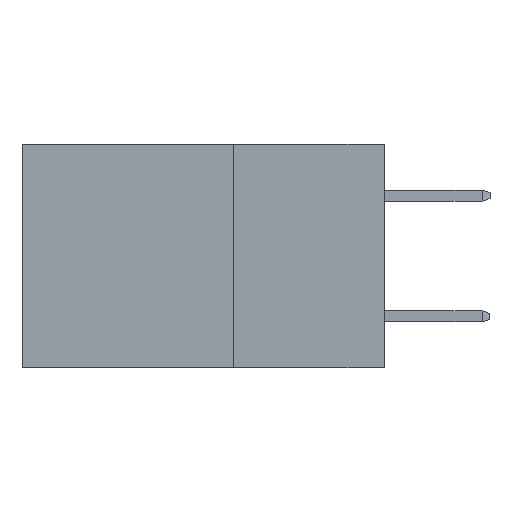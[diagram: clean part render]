
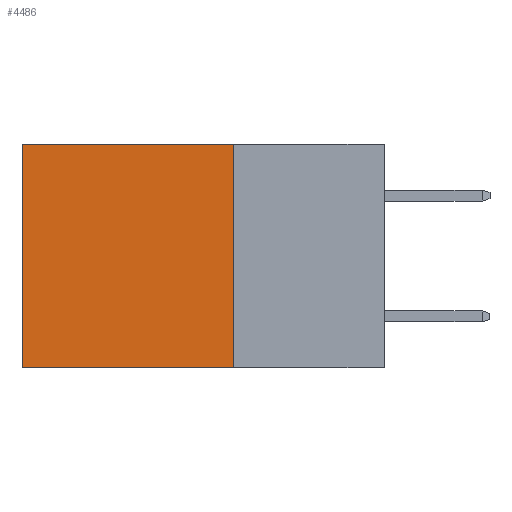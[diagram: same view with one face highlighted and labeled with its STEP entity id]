
A CAD part, left-side view. The second image highlights one B-rep face of the part: STEP entity #4486.
In plain terms, the highlighted planar face has unit normal (-1, 0, 0).
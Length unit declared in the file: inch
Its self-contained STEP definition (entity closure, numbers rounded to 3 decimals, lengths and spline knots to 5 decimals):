
#192 = LINE ( 'NONE', #7564, #5779 ) ;
#226 = VERTEX_POINT ( 'NONE', #15000 ) ;
#318 = LINE ( 'NONE', #11781, #12162 ) ;
#362 = ORIENTED_EDGE ( 'NONE', *, *, #3451, .F. ) ;
#821 = ORIENTED_EDGE ( 'NONE', *, *, #5099, .T. ) ;
#1122 = AXIS2_PLACEMENT_3D ( 'NONE', #11481, #11484, #8219 ) ;
#1388 = CARTESIAN_POINT ( 'NONE',  ( 0.298, 0.6, -0.37 ) ) ;
#1600 = DIRECTION ( 'NONE',  ( 0., 0., -1. ) ) ;
#1629 = DIRECTION ( 'NONE',  ( 0., 1., 0. ) ) ;
#2993 = VERTEX_POINT ( 'NONE', #5048 ) ;
#3451 = EDGE_CURVE ( 'NONE', #226, #10245, #6701, .T. ) ;
#4212 = FACE_OUTER_BOUND ( 'NONE', #6698, .T. ) ;
#4276 = ORIENTED_EDGE ( 'NONE', *, *, #15210, .T. ) ;
#4344 = CARTESIAN_POINT ( 'NONE',  ( 0.298, 0.6, 0. ) ) ;
#4486 = ADVANCED_FACE ( 'NONE', ( #4212 ), #12796, .F. ) ;
#5048 = CARTESIAN_POINT ( 'NONE',  ( 0.298, 0.25, 0. ) ) ;
#5099 = EDGE_CURVE ( 'NONE', #2993, #13568, #318, .T. ) ;
#5779 = VECTOR ( 'NONE', #1600, 39.37008 ) ;
#6698 = EDGE_LOOP ( 'NONE', ( #4276, #362, #14843, #821 ) ) ;
#6701 = LINE ( 'NONE', #14735, #9824 ) ;
#7564 = CARTESIAN_POINT ( 'NONE',  ( 0.298, 0.6, 0. ) ) ;
#7876 = VECTOR ( 'NONE', #12480, 39.37008 ) ;
#8219 = DIRECTION ( 'NONE',  ( 0., 0., -1. ) ) ;
#8327 = EDGE_CURVE ( 'NONE', #2993, #226, #14438, .T. ) ;
#9824 = VECTOR ( 'NONE', #1629, 39.37008 ) ;
#10245 = VERTEX_POINT ( 'NONE', #1388 ) ;
#11481 = CARTESIAN_POINT ( 'NONE',  ( 0.298, 0.25, 0. ) ) ;
#11484 = DIRECTION ( 'NONE',  ( 1., 0., 0. ) ) ;
#11781 = CARTESIAN_POINT ( 'NONE',  ( 0.298, 0.25, 0. ) ) ;
#12162 = VECTOR ( 'NONE', #12814, 39.37008 ) ;
#12453 = CARTESIAN_POINT ( 'NONE',  ( 0.298, 0.25, 0. ) ) ;
#12480 = DIRECTION ( 'NONE',  ( 0., 0., -1. ) ) ;
#12796 = PLANE ( 'NONE',  #1122 ) ;
#12814 = DIRECTION ( 'NONE',  ( 0., 1., 0. ) ) ;
#13568 = VERTEX_POINT ( 'NONE', #4344 ) ;
#14438 = LINE ( 'NONE', #12453, #7876 ) ;
#14735 = CARTESIAN_POINT ( 'NONE',  ( 0.298, 0.25, -0.37 ) ) ;
#14843 = ORIENTED_EDGE ( 'NONE', *, *, #8327, .F. ) ;
#15000 = CARTESIAN_POINT ( 'NONE',  ( 0.298, 0.25, -0.37 ) ) ;
#15210 = EDGE_CURVE ( 'NONE', #13568, #10245, #192, .T. ) ;
